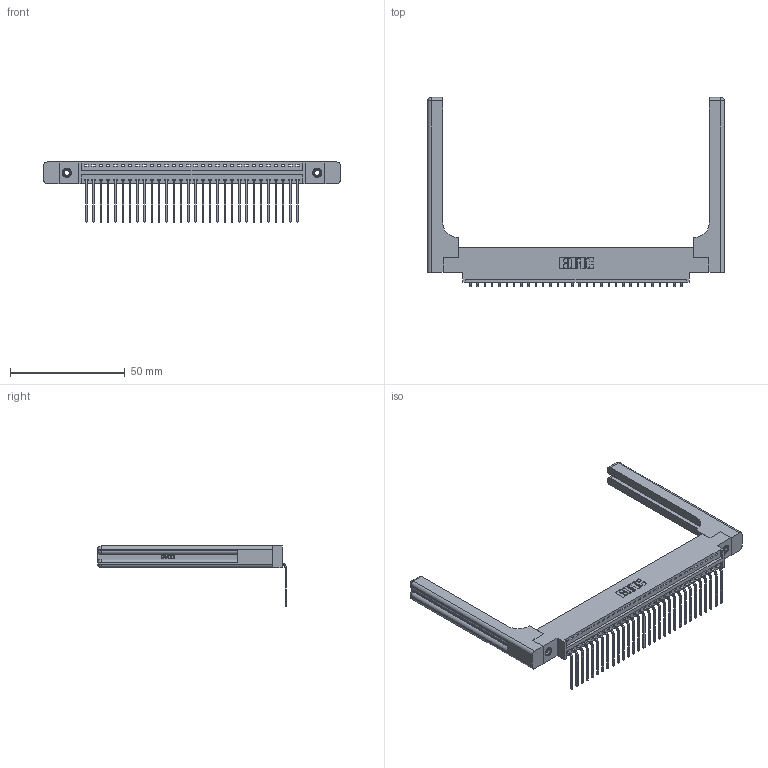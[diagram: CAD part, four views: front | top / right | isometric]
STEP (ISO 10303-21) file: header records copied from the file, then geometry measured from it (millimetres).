
FILE_DESCRIPTION (( 'STEP AP203' ), '1' );
FILE_NAME ('346-030-559-658.STEP', '2022-05-06T16:19:15', ( '' ), ( '' ), 'SwSTEP 2.0', 'SolidWorks 2020', '' );
FILE_SCHEMA (( 'CONFIG_CONTROL_DESIGN' ));
Length unit declared in the file: inch
Products named in the file (5): 346-030-559-658; 345-292-001_558 559 Tail - 1; 346-220-058_345-220-058; 345-250-001_345-250-001-102; 346 Part_0.170 Offset - 0.156 Dia-TH
Assembly tree (35 placements, depth 2):
  346-030-559-658
    346 Part_0.170 Offset - 0.156 Dia-TH
    345-292-001_558 559 Tail - 1  x30
    345-250-001_345-250-001-102  x2
    346-220-058_345-220-058  x2
Bounding box: 129.31 x 82.36 x 26.16 mm (x, y, z)
Volume: 19740.9 mm3; surface area: 21105.6 mm2
Topology: 35 solids, 35 shells, 2196 faces, 6503 edges, 4274 vertices
Faces by surface type: plane 1502, cylinder 634, bspline 36, cone 12, sphere 8, torus 4
Entity records: 26048 total; most frequent: CARTESIAN_POINT 5453, ORIENTED_EDGE 4212, DIRECTION 3754, EDGE_CURVE 2106, VECTOR 1762, LINE 1762, VERTEX_POINT 1394, AXIS2_PLACEMENT_3D 996
